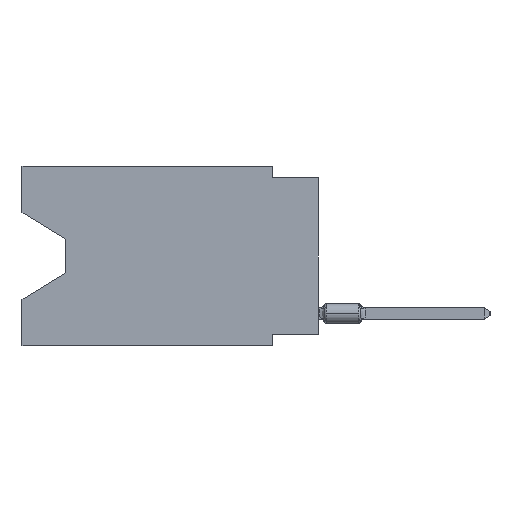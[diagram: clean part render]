
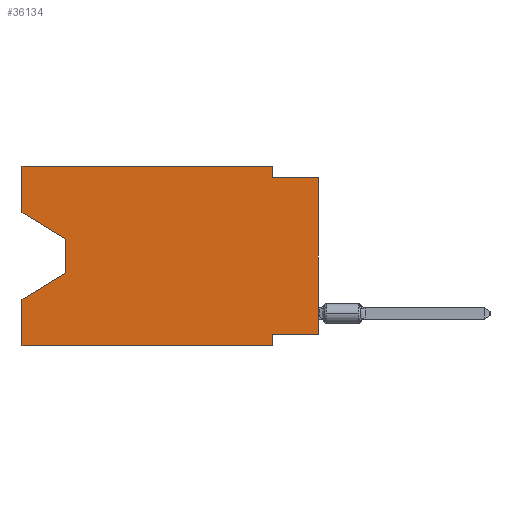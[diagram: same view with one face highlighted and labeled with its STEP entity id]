
A CAD part, left-side view. The second image highlights one B-rep face of the part: STEP entity #36134.
In plain terms, the highlighted planar face has unit normal (-1, 0, 0).
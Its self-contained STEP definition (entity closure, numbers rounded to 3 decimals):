
#4587 = VERTEX_POINT ( 'NONE', #37658 ) ;
#4765 = LINE ( 'NONE', #33985, #7362 ) ;
#5368 = AXIS2_PLACEMENT_3D ( 'NONE', #34372, #54345, #54014 ) ;
#5709 = EDGE_CURVE ( 'NONE', #30825, #9486, #8995, .T. ) ;
#6128 = DIRECTION ( 'NONE',  ( 0., -0.855, -0.519 ) ) ;
#7033 = VERTEX_POINT ( 'NONE', #45056 ) ;
#7362 = VECTOR ( 'NONE', #53950, 1000. ) ;
#8145 = LINE ( 'NONE', #24562, #44460 ) ;
#8553 = CARTESIAN_POINT ( 'NONE',  ( 0., 13.97, -4.013 ) ) ;
#8995 = LINE ( 'NONE', #19496, #36479 ) ;
#9235 = ORIENTED_EDGE ( 'NONE', *, *, #32575, .T. ) ;
#9486 = VERTEX_POINT ( 'NONE', #32179 ) ;
#10069 = LINE ( 'NONE', #45802, #10719 ) ;
#10302 = CARTESIAN_POINT ( 'NONE',  ( 0., 16.383, 0. ) ) ;
#10717 = DIRECTION ( 'NONE',  ( 0., 1., 0. ) ) ;
#10719 = VECTOR ( 'NONE', #6128, 1000. ) ;
#12144 = DIRECTION ( 'NONE',  ( 0., 0., 1. ) ) ;
#14958 = EDGE_CURVE ( 'NONE', #46234, #25209, #22640, .T. ) ;
#16497 = LINE ( 'NONE', #55851, #21330 ) ;
#16706 = EDGE_CURVE ( 'NONE', #25209, #43050, #58606, .T. ) ;
#16845 = VERTEX_POINT ( 'NONE', #45115 ) ;
#17771 = LINE ( 'NONE', #64882, #19548 ) ;
#17848 = CARTESIAN_POINT ( 'NONE',  ( 0., 16.383, -2.546 ) ) ;
#19496 = CARTESIAN_POINT ( 'NONE',  ( 0., 0., -0.635 ) ) ;
#19548 = VECTOR ( 'NONE', #32875, 1000. ) ;
#19695 = LINE ( 'NONE', #34147, #50608 ) ;
#20612 = VERTEX_POINT ( 'NONE', #31440 ) ;
#21330 = VECTOR ( 'NONE', #46318, 1000. ) ;
#22640 = LINE ( 'NONE', #52139, #27034 ) ;
#23259 = ORIENTED_EDGE ( 'NONE', *, *, #57525, .T. ) ;
#23527 = CARTESIAN_POINT ( 'NONE',  ( 0., 2.54, -9.906 ) ) ;
#24100 = DIRECTION ( 'NONE',  ( 0., -1., 0. ) ) ;
#24540 = FACE_OUTER_BOUND ( 'NONE', #53291, .T. ) ;
#24562 = CARTESIAN_POINT ( 'NONE',  ( 0., 16.383, 0. ) ) ;
#24884 = EDGE_CURVE ( 'NONE', #20612, #54939, #8145, .T. ) ;
#24915 = VECTOR ( 'NONE', #38913, 1000. ) ;
#25209 = VERTEX_POINT ( 'NONE', #10302 ) ;
#25510 = LINE ( 'NONE', #39587, #45905 ) ;
#25670 = ORIENTED_EDGE ( 'NONE', *, *, #24884, .F. ) ;
#26563 = CARTESIAN_POINT ( 'NONE',  ( 0., 16.383, -7.36 ) ) ;
#27034 = VECTOR ( 'NONE', #12144, 1000. ) ;
#28117 = ORIENTED_EDGE ( 'NONE', *, *, #39972, .T. ) ;
#30825 = VERTEX_POINT ( 'NONE', #50499 ) ;
#31440 = CARTESIAN_POINT ( 'NONE',  ( 0., 16.383, -9.906 ) ) ;
#32179 = CARTESIAN_POINT ( 'NONE',  ( 0., 0., -0.635 ) ) ;
#32451 = VECTOR ( 'NONE', #10717, 1000. ) ;
#32575 = EDGE_CURVE ( 'NONE', #20612, #37985, #25510, .T. ) ;
#32875 = DIRECTION ( 'NONE',  ( 0., 0., 1. ) ) ;
#33985 = CARTESIAN_POINT ( 'NONE',  ( 0., 2.54, -9.906 ) ) ;
#34147 = CARTESIAN_POINT ( 'NONE',  ( 0., 13.97, -4.013 ) ) ;
#34371 = EDGE_CURVE ( 'NONE', #4587, #7033, #40900, .T. ) ;
#34372 = CARTESIAN_POINT ( 'NONE',  ( 0., 16.383, 0. ) ) ;
#36134 = ADVANCED_FACE ( 'NONE', ( #24540 ), #48772, .F. ) ;
#36479 = VECTOR ( 'NONE', #24100, 1000. ) ;
#37658 = CARTESIAN_POINT ( 'NONE',  ( 0., 0., -9.271 ) ) ;
#37985 = VERTEX_POINT ( 'NONE', #23527 ) ;
#38088 = ORIENTED_EDGE ( 'NONE', *, *, #5709, .F. ) ;
#38727 = CARTESIAN_POINT ( 'NONE',  ( 0., 2.54, 0. ) ) ;
#38913 = DIRECTION ( 'NONE',  ( 0., -1., 0. ) ) ;
#39587 = CARTESIAN_POINT ( 'NONE',  ( 0., 16.383, -9.906 ) ) ;
#39756 = ORIENTED_EDGE ( 'NONE', *, *, #61662, .T. ) ;
#39972 = EDGE_CURVE ( 'NONE', #16845, #54939, #60868, .T. ) ;
#40900 = LINE ( 'NONE', #45806, #32451 ) ;
#41294 = EDGE_CURVE ( 'NONE', #7033, #37985, #4765, .T. ) ;
#42847 = VECTOR ( 'NONE', #54954, 1000. ) ;
#42896 = ORIENTED_EDGE ( 'NONE', *, *, #34371, .F. ) ;
#43050 = VERTEX_POINT ( 'NONE', #38727 ) ;
#43624 = ORIENTED_EDGE ( 'NONE', *, *, #56477, .T. ) ;
#44460 = VECTOR ( 'NONE', #64547, 1000. ) ;
#45056 = CARTESIAN_POINT ( 'NONE',  ( 0., 2.54, -9.271 ) ) ;
#45115 = CARTESIAN_POINT ( 'NONE',  ( 0., 13.97, -5.893 ) ) ;
#45319 = ORIENTED_EDGE ( 'NONE', *, *, #16706, .F. ) ;
#45610 = ORIENTED_EDGE ( 'NONE', *, *, #14958, .F. ) ;
#45802 = CARTESIAN_POINT ( 'NONE',  ( 0., 16.383, -2.546 ) ) ;
#45806 = CARTESIAN_POINT ( 'NONE',  ( 0., 0., -9.271 ) ) ;
#45905 = VECTOR ( 'NONE', #55331, 1000. ) ;
#46234 = VERTEX_POINT ( 'NONE', #17848 ) ;
#46318 = DIRECTION ( 'NONE',  ( 0., 0., -1. ) ) ;
#46435 = EDGE_CURVE ( 'NONE', #43050, #30825, #16497, .T. ) ;
#48208 = ORIENTED_EDGE ( 'NONE', *, *, #46435, .F. ) ;
#48772 = PLANE ( 'NONE',  #5368 ) ;
#50156 = VERTEX_POINT ( 'NONE', #8553 ) ;
#50351 = CARTESIAN_POINT ( 'NONE',  ( 0., 13.97, -5.893 ) ) ;
#50499 = CARTESIAN_POINT ( 'NONE',  ( 0., 2.54, -0.635 ) ) ;
#50608 = VECTOR ( 'NONE', #64617, 1000. ) ;
#52139 = CARTESIAN_POINT ( 'NONE',  ( 0., 16.383, 0. ) ) ;
#53037 = ORIENTED_EDGE ( 'NONE', *, *, #41294, .F. ) ;
#53291 = EDGE_LOOP ( 'NONE', ( #43624, #23259, #28117, #25670, #9235, #53037, #42896, #39756, #38088, #48208, #45319, #45610 ) ) ;
#53950 = DIRECTION ( 'NONE',  ( 0., 0., -1. ) ) ;
#54014 = DIRECTION ( 'NONE',  ( 0., 0., -1. ) ) ;
#54345 = DIRECTION ( 'NONE',  ( 1., 0., 0. ) ) ;
#54939 = VERTEX_POINT ( 'NONE', #26563 ) ;
#54954 = DIRECTION ( 'NONE',  ( 0., 0.855, -0.519 ) ) ;
#55331 = DIRECTION ( 'NONE',  ( 0., -1., 0. ) ) ;
#55851 = CARTESIAN_POINT ( 'NONE',  ( 0., 2.54, 0. ) ) ;
#56477 = EDGE_CURVE ( 'NONE', #46234, #50156, #10069, .T. ) ;
#57525 = EDGE_CURVE ( 'NONE', #50156, #16845, #19695, .T. ) ;
#58273 = CARTESIAN_POINT ( 'NONE',  ( 0., 16.383, 0. ) ) ;
#58606 = LINE ( 'NONE', #58273, #24915 ) ;
#60868 = LINE ( 'NONE', #50351, #42847 ) ;
#61662 = EDGE_CURVE ( 'NONE', #4587, #9486, #17771, .T. ) ;
#64547 = DIRECTION ( 'NONE',  ( 0., 0., 1. ) ) ;
#64617 = DIRECTION ( 'NONE',  ( 0., 0., -1. ) ) ;
#64882 = CARTESIAN_POINT ( 'NONE',  ( 0., 0., 0. ) ) ;
